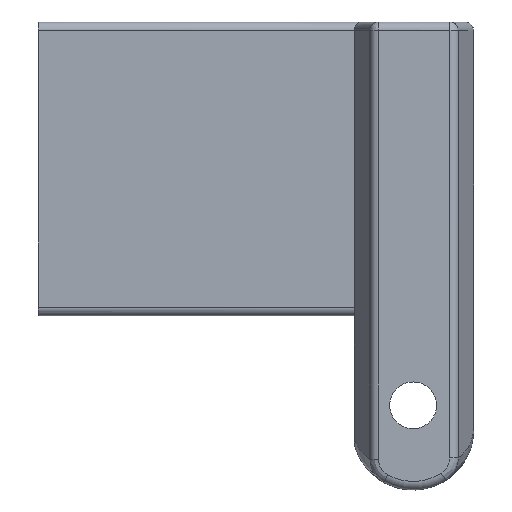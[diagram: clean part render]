
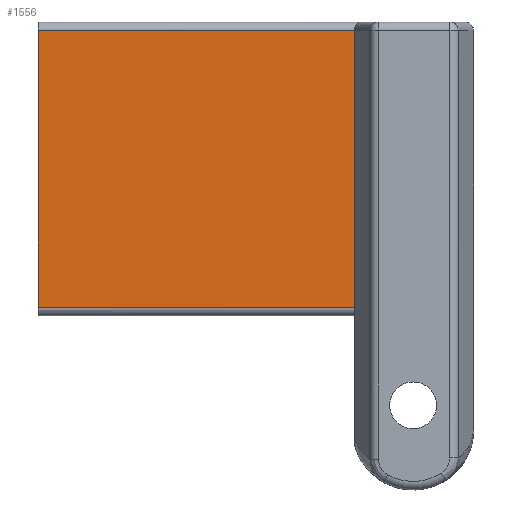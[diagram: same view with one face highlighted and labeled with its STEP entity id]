
A CAD part, front view. The second image highlights one B-rep face of the part: STEP entity #1556.
In plain terms, the highlighted planar face has unit normal (0, -1, 0).
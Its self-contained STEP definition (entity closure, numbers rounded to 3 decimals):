
#107 = LINE ( 'NONE', #471, #134 ) ;
#134 = VECTOR ( 'NONE', #852, 1000. ) ;
#181 = LINE ( 'NONE', #1518, #1367 ) ;
#190 = EDGE_CURVE ( 'NONE', #1063, #232, #848, .T. ) ;
#194 = ORIENTED_EDGE ( 'NONE', *, *, #190, .F. ) ;
#232 = VERTEX_POINT ( 'NONE', #907 ) ;
#239 = FACE_OUTER_BOUND ( 'NONE', #684, .T. ) ;
#251 = DIRECTION ( 'NONE',  ( 1., 0., 0. ) ) ;
#263 = CARTESIAN_POINT ( 'NONE',  ( -219.205, 17.562, -16.057 ) ) ;
#282 = VERTEX_POINT ( 'NONE', #764 ) ;
#372 = LINE ( 'NONE', #1226, #847 ) ;
#382 = DIRECTION ( 'NONE',  ( -1., 0., 0. ) ) ;
#431 = CARTESIAN_POINT ( 'NONE',  ( -223.381, 17.562, -4.772 ) ) ;
#471 = CARTESIAN_POINT ( 'NONE',  ( -255.316, 17.562, -2.025 ) ) ;
#494 = VERTEX_POINT ( 'NONE', #828 ) ;
#516 = ORIENTED_EDGE ( 'NONE', *, *, #787, .F. ) ;
#524 = DIRECTION ( 'NONE',  ( 0., 0., -1. ) ) ;
#605 = DIRECTION ( 'NONE',  ( 0., 0., 1. ) ) ;
#624 = LINE ( 'NONE', #997, #1502 ) ;
#630 = CARTESIAN_POINT ( 'NONE',  ( -219.205, 17.562, 16.503 ) ) ;
#642 = ORIENTED_EDGE ( 'NONE', *, *, #985, .F. ) ;
#684 = EDGE_LOOP ( 'NONE', ( #924, #194, #516, #1033, #1100, #642 ) ) ;
#687 = VECTOR ( 'NONE', #382, 1000. ) ;
#730 = DIRECTION ( 'NONE',  ( 1., 0., 0. ) ) ;
#751 = EDGE_CURVE ( 'NONE', #494, #1014, #372, .T. ) ;
#764 = CARTESIAN_POINT ( 'NONE',  ( -255.316, 17.562, 16.503 ) ) ;
#787 = EDGE_CURVE ( 'NONE', #494, #1063, #1080, .T. ) ;
#828 = CARTESIAN_POINT ( 'NONE',  ( -219.21, 17.562, -16.057 ) ) ;
#847 = VECTOR ( 'NONE', #730, 1000. ) ;
#848 = LINE ( 'NONE', #1402, #687 ) ;
#852 = DIRECTION ( 'NONE',  ( 0., 0., -1. ) ) ;
#857 = EDGE_CURVE ( 'NONE', #282, #232, #107, .T. ) ;
#907 = CARTESIAN_POINT ( 'NONE',  ( -255.316, 17.562, -15.057 ) ) ;
#911 = DIRECTION ( 'NONE',  ( 1., 0., 0. ) ) ;
#917 = CARTESIAN_POINT ( 'NONE',  ( -219.21, 17.562, -15.057 ) ) ;
#924 = ORIENTED_EDGE ( 'NONE', *, *, #857, .T. ) ;
#959 = AXIS2_PLACEMENT_3D ( 'NONE', #431, #1426, #911 ) ;
#985 = EDGE_CURVE ( 'NONE', #282, #1188, #624, .T. ) ;
#997 = CARTESIAN_POINT ( 'NONE',  ( -217.689, 17.562, 16.503 ) ) ;
#1001 = EDGE_CURVE ( 'NONE', #1188, #1014, #181, .T. ) ;
#1014 = VERTEX_POINT ( 'NONE', #263 ) ;
#1033 = ORIENTED_EDGE ( 'NONE', *, *, #751, .T. ) ;
#1063 = VERTEX_POINT ( 'NONE', #917 ) ;
#1080 = LINE ( 'NONE', #1343, #1590 ) ;
#1100 = ORIENTED_EDGE ( 'NONE', *, *, #1001, .F. ) ;
#1188 = VERTEX_POINT ( 'NONE', #630 ) ;
#1226 = CARTESIAN_POINT ( 'NONE',  ( -226.401, 17.562, -16.057 ) ) ;
#1302 = PLANE ( 'NONE',  #959 ) ;
#1343 = CARTESIAN_POINT ( 'NONE',  ( -219.21, 17.562, -7.363 ) ) ;
#1367 = VECTOR ( 'NONE', #524, 1000. ) ;
#1402 = CARTESIAN_POINT ( 'NONE',  ( -226.401, 17.562, -15.057 ) ) ;
#1426 = DIRECTION ( 'NONE',  ( 0., -1., 0. ) ) ;
#1502 = VECTOR ( 'NONE', #251, 1000. ) ;
#1518 = CARTESIAN_POINT ( 'NONE',  ( -219.205, 17.562, -3.432 ) ) ;
#1556 = ADVANCED_FACE ( 'NONE', ( #239 ), #1302, .T. ) ;
#1590 = VECTOR ( 'NONE', #605, 1000. ) ;
